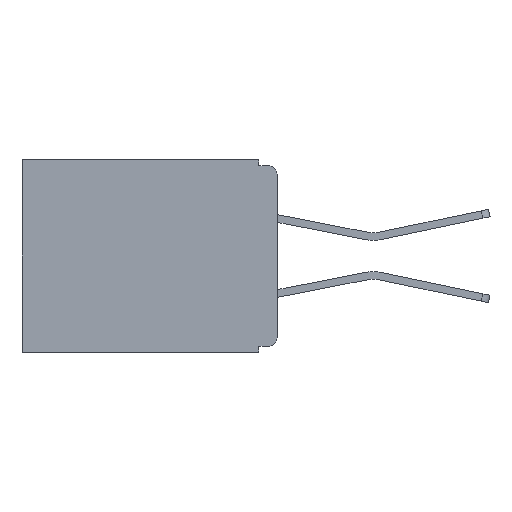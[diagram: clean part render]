
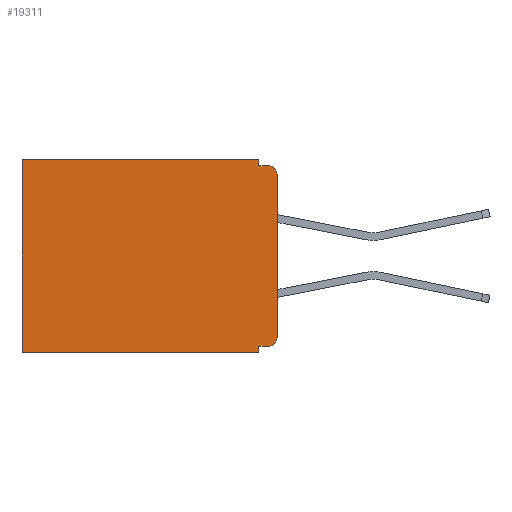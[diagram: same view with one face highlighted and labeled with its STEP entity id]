
A CAD part, left-side view. The second image highlights one B-rep face of the part: STEP entity #19311.
In plain terms, the highlighted planar face has unit normal (-1, 0, 0).
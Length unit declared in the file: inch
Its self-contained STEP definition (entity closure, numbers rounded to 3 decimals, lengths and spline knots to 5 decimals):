
#222 = CARTESIAN_POINT ( 'NONE',  ( 0.3, 0., -0.305 ) ) ;
#435 = CARTESIAN_POINT ( 'NONE',  ( 0.3, 0.031, 0. ) ) ;
#798 = ORIENTED_EDGE ( 'NONE', *, *, #6855, .F. ) ;
#1189 = VERTEX_POINT ( 'NONE', #5204 ) ;
#1300 = VERTEX_POINT ( 'NONE', #26697 ) ;
#2248 = VERTEX_POINT ( 'NONE', #3903 ) ;
#2810 = LINE ( 'NONE', #7854, #13642 ) ;
#3020 = VERTEX_POINT ( 'NONE', #17845 ) ;
#3177 = AXIS2_PLACEMENT_3D ( 'NONE', #3826, #18994, #6041 ) ;
#3276 = CARTESIAN_POINT ( 'NONE',  ( 0.3, 0., -0.32 ) ) ;
#3819 = DIRECTION ( 'NONE',  ( 0., 0., -1. ) ) ;
#3826 = CARTESIAN_POINT ( 'NONE',  ( 0.3, 0.015, -0.025 ) ) ;
#3903 = CARTESIAN_POINT ( 'NONE',  ( 0.3, 0.031, -0.32 ) ) ;
#3967 = VECTOR ( 'NONE', #22213, 39.37008 ) ;
#4133 = VERTEX_POINT ( 'NONE', #23050 ) ;
#4171 = VERTEX_POINT ( 'NONE', #22714 ) ;
#4288 = DIRECTION ( 'NONE',  ( 0., 1., 0. ) ) ;
#5204 = CARTESIAN_POINT ( 'NONE',  ( 0.3, 0.015, -0.01 ) ) ;
#5831 = LINE ( 'NONE', #10337, #10869 ) ;
#6041 = DIRECTION ( 'NONE',  ( 0., 0., -1. ) ) ;
#6104 = VERTEX_POINT ( 'NONE', #7518 ) ;
#6855 = EDGE_CURVE ( 'NONE', #11555, #10012, #2810, .T. ) ;
#7131 = ORIENTED_EDGE ( 'NONE', *, *, #21526, .F. ) ;
#7239 = VECTOR ( 'NONE', #26865, 39.37008 ) ;
#7518 = CARTESIAN_POINT ( 'NONE',  ( 0.3, 0.437, 0. ) ) ;
#7854 = CARTESIAN_POINT ( 'NONE',  ( 0.3, 0., -0.33 ) ) ;
#8382 = VECTOR ( 'NONE', #19891, 39.37008 ) ;
#8395 = VECTOR ( 'NONE', #3819, 39.37008 ) ;
#8472 = LINE ( 'NONE', #3276, #13538 ) ;
#8755 = VECTOR ( 'NONE', #24354, 39.37008 ) ;
#9178 = CARTESIAN_POINT ( 'NONE',  ( 0.3, 0., -0.33 ) ) ;
#9664 = EDGE_LOOP ( 'NONE', ( #798, #27247, #27918, #15504, #10495, #24047, #7131, #14804, #23840, #25545 ) ) ;
#9901 = EDGE_CURVE ( 'NONE', #2248, #4171, #19957, .T. ) ;
#10012 = VERTEX_POINT ( 'NONE', #222 ) ;
#10180 = CARTESIAN_POINT ( 'NONE',  ( 0.3, 0., -0.33 ) ) ;
#10337 = CARTESIAN_POINT ( 'NONE',  ( 0.3, 0., 0. ) ) ;
#10495 = ORIENTED_EDGE ( 'NONE', *, *, #12996, .T. ) ;
#10525 = AXIS2_PLACEMENT_3D ( 'NONE', #10180, #25312, #12321 ) ;
#10773 = CARTESIAN_POINT ( 'NONE',  ( 0.3, 0.015, -0.305 ) ) ;
#10869 = VECTOR ( 'NONE', #4288, 39.37008 ) ;
#11122 = CIRCLE ( 'NONE', #26501, 0.015 ) ;
#11346 = EDGE_CURVE ( 'NONE', #4133, #3020, #27594, .T. ) ;
#11555 = VERTEX_POINT ( 'NONE', #27015 ) ;
#12190 = DIRECTION ( 'NONE',  ( 0., 0., -1. ) ) ;
#12321 = DIRECTION ( 'NONE',  ( 0., 0., -1. ) ) ;
#12916 = DIRECTION ( 'NONE',  ( 0., 0., -1. ) ) ;
#12996 = EDGE_CURVE ( 'NONE', #4133, #6104, #5831, .T. ) ;
#13538 = VECTOR ( 'NONE', #14068, 39.37008 ) ;
#13642 = VECTOR ( 'NONE', #12190, 39.37008 ) ;
#14068 = DIRECTION ( 'NONE',  ( 0., 1., 0. ) ) ;
#14144 = LINE ( 'NONE', #15511, #8382 ) ;
#14610 = CARTESIAN_POINT ( 'NONE',  ( 0.3, 0.031, -0.33 ) ) ;
#14619 = EDGE_CURVE ( 'NONE', #1300, #10012, #11122, .T. ) ;
#14804 = ORIENTED_EDGE ( 'NONE', *, *, #9901, .F. ) ;
#15504 = ORIENTED_EDGE ( 'NONE', *, *, #11346, .F. ) ;
#15511 = CARTESIAN_POINT ( 'NONE',  ( 0.3, 0., -0.01 ) ) ;
#16109 = CARTESIAN_POINT ( 'NONE',  ( 0.3, 0.437, -0.33 ) ) ;
#17506 = VERTEX_POINT ( 'NONE', #21076 ) ;
#17522 = EDGE_CURVE ( 'NONE', #11555, #1189, #22133, .T. ) ;
#17845 = CARTESIAN_POINT ( 'NONE',  ( 0.3, 0.031, -0.01 ) ) ;
#18756 = LINE ( 'NONE', #16109, #7239 ) ;
#18994 = DIRECTION ( 'NONE',  ( -1., 0., 0. ) ) ;
#19081 = FACE_OUTER_BOUND ( 'NONE', #9664, .T. ) ;
#19311 = ADVANCED_FACE ( 'NONE', ( #19081 ), #20989, .F. ) ;
#19645 = LINE ( 'NONE', #9178, #8755 ) ;
#19891 = DIRECTION ( 'NONE',  ( 0., -1., 0. ) ) ;
#19957 = LINE ( 'NONE', #14610, #8395 ) ;
#20466 = EDGE_CURVE ( 'NONE', #1300, #2248, #8472, .T. ) ;
#20989 = PLANE ( 'NONE',  #10525 ) ;
#21076 = CARTESIAN_POINT ( 'NONE',  ( 0.3, 0.437, -0.33 ) ) ;
#21526 = EDGE_CURVE ( 'NONE', #4171, #17506, #19645, .T. ) ;
#22133 = CIRCLE ( 'NONE', #3177, 0.015 ) ;
#22213 = DIRECTION ( 'NONE',  ( 0., 0., -1. ) ) ;
#22714 = CARTESIAN_POINT ( 'NONE',  ( 0.3, 0.031, -0.33 ) ) ;
#23050 = CARTESIAN_POINT ( 'NONE',  ( 0.3, 0.031, 0. ) ) ;
#23840 = ORIENTED_EDGE ( 'NONE', *, *, #20466, .F. ) ;
#24047 = ORIENTED_EDGE ( 'NONE', *, *, #24368, .T. ) ;
#24354 = DIRECTION ( 'NONE',  ( 0., 1., 0. ) ) ;
#24368 = EDGE_CURVE ( 'NONE', #6104, #17506, #18756, .T. ) ;
#25312 = DIRECTION ( 'NONE',  ( 1., 0., 0. ) ) ;
#25545 = ORIENTED_EDGE ( 'NONE', *, *, #14619, .T. ) ;
#25896 = DIRECTION ( 'NONE',  ( -1., 0., 0. ) ) ;
#26501 = AXIS2_PLACEMENT_3D ( 'NONE', #10773, #25896, #12916 ) ;
#26697 = CARTESIAN_POINT ( 'NONE',  ( 0.3, 0.015, -0.32 ) ) ;
#26865 = DIRECTION ( 'NONE',  ( 0., 0., -1. ) ) ;
#27015 = CARTESIAN_POINT ( 'NONE',  ( 0.3, 0., -0.025 ) ) ;
#27247 = ORIENTED_EDGE ( 'NONE', *, *, #17522, .T. ) ;
#27594 = LINE ( 'NONE', #435, #3967 ) ;
#27606 = EDGE_CURVE ( 'NONE', #3020, #1189, #14144, .T. ) ;
#27918 = ORIENTED_EDGE ( 'NONE', *, *, #27606, .F. ) ;
